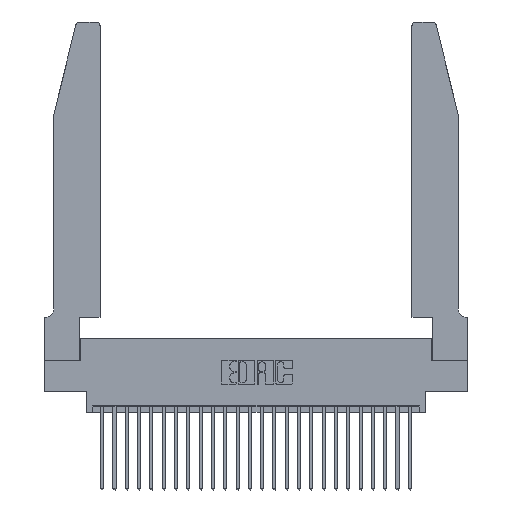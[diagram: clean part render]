
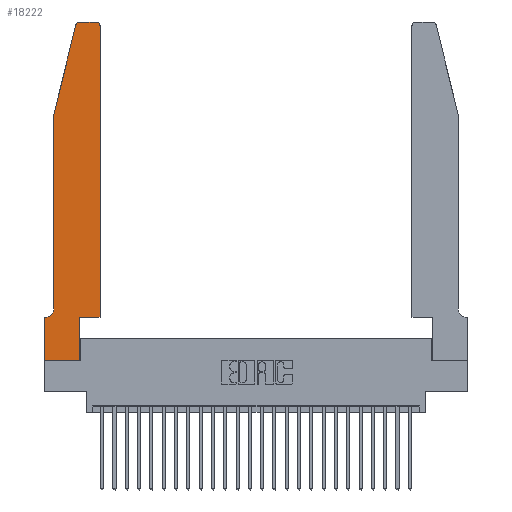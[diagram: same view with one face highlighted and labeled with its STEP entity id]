
A CAD part, top view. The second image highlights one B-rep face of the part: STEP entity #18222.
In plain terms, the highlighted planar face has unit normal (0, 0, 1).
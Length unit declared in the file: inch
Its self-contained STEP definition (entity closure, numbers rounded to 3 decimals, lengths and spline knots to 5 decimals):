
#422 = VERTEX_POINT ( 'NONE', #1332 ) ;
#1332 = CARTESIAN_POINT ( 'NONE',  ( 0.284, 2.75, 0.37 ) ) ;
#1363 = CARTESIAN_POINT ( 'NONE',  ( 0.2865, 0.35, 0.37 ) ) ;
#1729 = VERTEX_POINT ( 'NONE', #20696 ) ;
#2015 = VECTOR ( 'NONE', #21506, 39.37008 ) ;
#2732 = EDGE_CURVE ( 'NONE', #4046, #1729, #21133, .T. ) ;
#2902 = EDGE_CURVE ( 'NONE', #17904, #422, #12352, .T. ) ;
#2924 = CIRCLE ( 'NONE', #6068, 0.03 ) ;
#3892 = AXIS2_PLACEMENT_3D ( 'NONE', #17435, #4672, #19507 ) ;
#4046 = VERTEX_POINT ( 'NONE', #17506 ) ;
#4604 = EDGE_CURVE ( 'NONE', #7563, #4046, #17508, .T. ) ;
#4632 = CARTESIAN_POINT ( 'NONE',  ( 0.4505, 0.35, 0.37 ) ) ;
#4672 = DIRECTION ( 'NONE',  ( 0., 0., 1. ) ) ;
#4826 = CARTESIAN_POINT ( 'NONE',  ( 0.2865, 0.35, 0.37 ) ) ;
#4854 = VECTOR ( 'NONE', #26394, 39.37008 ) ;
#6068 = AXIS2_PLACEMENT_3D ( 'NONE', #25460, #13159, #14888 ) ;
#6252 = CARTESIAN_POINT ( 'NONE',  ( 0.4205, 2.75, 0.37 ) ) ;
#6521 = VERTEX_POINT ( 'NONE', #22414 ) ;
#6732 = DIRECTION ( 'NONE',  ( 0., 0., -1. ) ) ;
#7183 = ORIENTED_EDGE ( 'NONE', *, *, #8146, .T. ) ;
#7278 = AXIS2_PLACEMENT_3D ( 'NONE', #19392, #6732, #21423 ) ;
#7342 = ORIENTED_EDGE ( 'NONE', *, *, #18666, .T. ) ;
#7563 = VERTEX_POINT ( 'NONE', #15671 ) ;
#8050 = LINE ( 'NONE', #21067, #24658 ) ;
#8056 = CARTESIAN_POINT ( 'NONE',  ( 0.0755, 2., 0.37 ) ) ;
#8105 = DIRECTION ( 'NONE',  ( -1., 0., 0. ) ) ;
#8146 = EDGE_CURVE ( 'NONE', #20786, #22956, #18674, .T. ) ;
#8377 = CARTESIAN_POINT ( 'NONE',  ( 0.25487, 2.72718, 0.37 ) ) ;
#9184 = DIRECTION ( 'NONE',  ( 1., 0., 0. ) ) ;
#9508 = PLANE ( 'NONE',  #17821 ) ;
#10934 = VECTOR ( 'NONE', #8105, 39.37008 ) ;
#11401 = EDGE_LOOP ( 'NONE', ( #24146, #16722, #11594, #21088, #26448, #15221, #18913, #18973, #22668, #7183, #18100, #7342 ) ) ;
#11594 = ORIENTED_EDGE ( 'NONE', *, *, #20035, .T. ) ;
#11616 = LINE ( 'NONE', #22723, #10934 ) ;
#11662 = DIRECTION ( 'NONE',  ( 0., 0., 1. ) ) ;
#11913 = VECTOR ( 'NONE', #25241, 39.37008 ) ;
#11947 = CARTESIAN_POINT ( 'NONE',  ( 0.0755, 2., 0.37 ) ) ;
#12352 = LINE ( 'NONE', #26629, #22089 ) ;
#12354 = CARTESIAN_POINT ( 'NONE',  ( 0.4505, 2.72, 0.37 ) ) ;
#12631 = VERTEX_POINT ( 'NONE', #8377 ) ;
#13159 = DIRECTION ( 'NONE',  ( 0., 0., 1. ) ) ;
#13419 = DIRECTION ( 'NONE',  ( -1., 0., 0. ) ) ;
#14888 = DIRECTION ( 'NONE',  ( 1., 0., 0. ) ) ;
#14941 = VERTEX_POINT ( 'NONE', #19370 ) ;
#15044 = VECTOR ( 'NONE', #20573, 39.37008 ) ;
#15221 = ORIENTED_EDGE ( 'NONE', *, *, #25083, .T. ) ;
#15671 = CARTESIAN_POINT ( 'NONE',  ( 0., 0.35, 0.37 ) ) ;
#15777 = CARTESIAN_POINT ( 'NONE',  ( 0.4505, 0.35, 0.37 ) ) ;
#16546 = VERTEX_POINT ( 'NONE', #8056 ) ;
#16722 = ORIENTED_EDGE ( 'NONE', *, *, #17422, .T. ) ;
#17422 = EDGE_CURVE ( 'NONE', #422, #12631, #2924, .T. ) ;
#17435 = CARTESIAN_POINT ( 'NONE',  ( 0.4205, 2.72, 0.37 ) ) ;
#17506 = CARTESIAN_POINT ( 'NONE',  ( 0., 0., 0.37 ) ) ;
#17508 = LINE ( 'NONE', #27203, #11913 ) ;
#17821 = AXIS2_PLACEMENT_3D ( 'NONE', #24061, #11662, #26135 ) ;
#17903 = EDGE_CURVE ( 'NONE', #16546, #14941, #8050, .T. ) ;
#17904 = VERTEX_POINT ( 'NONE', #6252 ) ;
#18100 = ORIENTED_EDGE ( 'NONE', *, *, #25949, .T. ) ;
#18222 = ADVANCED_FACE ( 'NONE', ( #27190 ), #9508, .T. ) ;
#18288 = CIRCLE ( 'NONE', #7278, 0.07 ) ;
#18666 = EDGE_CURVE ( 'NONE', #20824, #17904, #27170, .T. ) ;
#18674 = LINE ( 'NONE', #19670, #25345 ) ;
#18913 = ORIENTED_EDGE ( 'NONE', *, *, #4604, .T. ) ;
#18973 = ORIENTED_EDGE ( 'NONE', *, *, #2732, .T. ) ;
#19370 = CARTESIAN_POINT ( 'NONE',  ( 0.0755, 0.42, 0.37 ) ) ;
#19392 = CARTESIAN_POINT ( 'NONE',  ( 0.0055, 0.42, 0.37 ) ) ;
#19507 = DIRECTION ( 'NONE',  ( 1., 0., 0. ) ) ;
#19670 = CARTESIAN_POINT ( 'NONE',  ( 0.4505, 0.35, 0.37 ) ) ;
#20035 = EDGE_CURVE ( 'NONE', #12631, #16546, #27093, .T. ) ;
#20573 = DIRECTION ( 'NONE',  ( 1., 0., 0. ) ) ;
#20696 = CARTESIAN_POINT ( 'NONE',  ( 0.2865, 0., 0.37 ) ) ;
#20786 = VERTEX_POINT ( 'NONE', #1363 ) ;
#20824 = VERTEX_POINT ( 'NONE', #12354 ) ;
#21067 = CARTESIAN_POINT ( 'NONE',  ( 0.0755, 2., 0.37 ) ) ;
#21088 = ORIENTED_EDGE ( 'NONE', *, *, #17903, .T. ) ;
#21133 = LINE ( 'NONE', #22736, #15044 ) ;
#21423 = DIRECTION ( 'NONE',  ( -1., 0., 0. ) ) ;
#21506 = DIRECTION ( 'NONE',  ( 0., 1., 0. ) ) ;
#21985 = VECTOR ( 'NONE', #25794, 39.37008 ) ;
#22089 = VECTOR ( 'NONE', #13419, 39.37008 ) ;
#22414 = CARTESIAN_POINT ( 'NONE',  ( 0.0055, 0.35, 0.37 ) ) ;
#22620 = LINE ( 'NONE', #4826, #21985 ) ;
#22668 = ORIENTED_EDGE ( 'NONE', *, *, #26007, .T. ) ;
#22723 = CARTESIAN_POINT ( 'NONE',  ( 0.0755, 0.35, 0.37 ) ) ;
#22736 = CARTESIAN_POINT ( 'NONE',  ( 0., 0., 0.37 ) ) ;
#22956 = VERTEX_POINT ( 'NONE', #15777 ) ;
#23882 = LINE ( 'NONE', #4632, #2015 ) ;
#23956 = EDGE_CURVE ( 'NONE', #14941, #6521, #18288, .T. ) ;
#24061 = CARTESIAN_POINT ( 'NONE',  ( 0., 0.35, 0.37 ) ) ;
#24146 = ORIENTED_EDGE ( 'NONE', *, *, #2902, .T. ) ;
#24658 = VECTOR ( 'NONE', #25150, 39.37008 ) ;
#25083 = EDGE_CURVE ( 'NONE', #6521, #7563, #11616, .T. ) ;
#25150 = DIRECTION ( 'NONE',  ( 0., -1., 0. ) ) ;
#25241 = DIRECTION ( 'NONE',  ( 0., -1., 0. ) ) ;
#25345 = VECTOR ( 'NONE', #9184, 39.37008 ) ;
#25460 = CARTESIAN_POINT ( 'NONE',  ( 0.284, 2.72, 0.37 ) ) ;
#25794 = DIRECTION ( 'NONE',  ( 0., 1., 0. ) ) ;
#25949 = EDGE_CURVE ( 'NONE', #22956, #20824, #23882, .T. ) ;
#26007 = EDGE_CURVE ( 'NONE', #1729, #20786, #22620, .T. ) ;
#26135 = DIRECTION ( 'NONE',  ( 1., 0., 0. ) ) ;
#26394 = DIRECTION ( 'NONE',  ( -0.239, -0.971, 0. ) ) ;
#26448 = ORIENTED_EDGE ( 'NONE', *, *, #23956, .T. ) ;
#26629 = CARTESIAN_POINT ( 'NONE',  ( 0.2605, 2.75, 0.37 ) ) ;
#27093 = LINE ( 'NONE', #11947, #4854 ) ;
#27170 = CIRCLE ( 'NONE', #3892, 0.03 ) ;
#27190 = FACE_OUTER_BOUND ( 'NONE', #11401, .T. ) ;
#27203 = CARTESIAN_POINT ( 'NONE',  ( 0., 0., 0.37 ) ) ;
